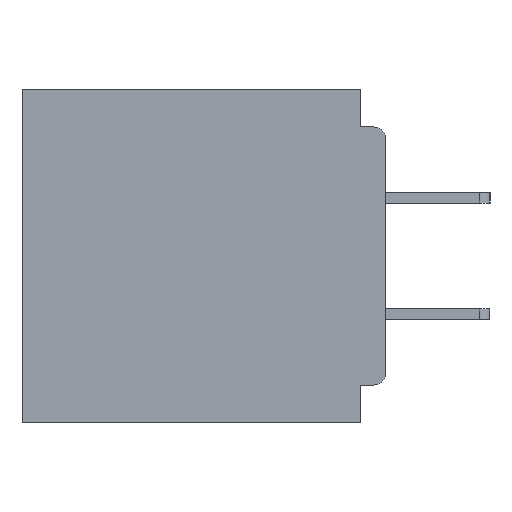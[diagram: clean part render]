
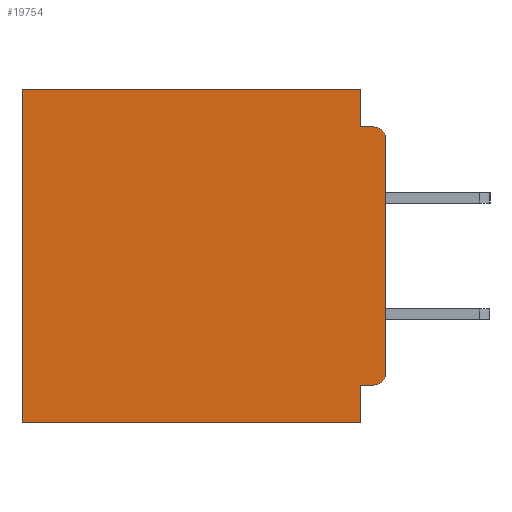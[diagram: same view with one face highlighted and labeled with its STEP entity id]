
A CAD part, left-side view. The second image highlights one B-rep face of the part: STEP entity #19754.
In plain terms, the highlighted planar face has unit normal (-1, 0, 0).
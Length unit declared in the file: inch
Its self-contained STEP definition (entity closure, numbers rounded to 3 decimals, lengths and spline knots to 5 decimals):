
#26 = VECTOR ( 'NONE', #40239, 39.37008 ) ;
#572 = CARTESIAN_POINT ( 'NONE',  ( 0.3, 0., 0. ) ) ;
#896 = CARTESIAN_POINT ( 'NONE',  ( 0.3, 0.437, -0.4 ) ) ;
#951 = CARTESIAN_POINT ( 'NONE',  ( 0.3, 0.437, -0.4 ) ) ;
#1415 = DIRECTION ( 'NONE',  ( 0., 0., -1. ) ) ;
#1472 = LINE ( 'NONE', #30982, #26 ) ;
#1840 = DIRECTION ( 'NONE',  ( -1., 0., 0. ) ) ;
#1983 = LINE ( 'NONE', #951, #49897 ) ;
#2817 = VERTEX_POINT ( 'NONE', #29447 ) ;
#5861 = EDGE_LOOP ( 'NONE', ( #54353, #28325, #51363, #54717, #31887, #22470, #36258, #59076, #18633, #49215 ) ) ;
#6317 = EDGE_CURVE ( 'NONE', #19578, #14118, #29886, .T. ) ;
#6645 = VECTOR ( 'NONE', #54614, 39.37008 ) ;
#8592 = CARTESIAN_POINT ( 'NONE',  ( 0.3, 0.437, 0. ) ) ;
#9813 = CIRCLE ( 'NONE', #55843, 0.015 ) ;
#11366 = EDGE_CURVE ( 'NONE', #14173, #22456, #1472, .T. ) ;
#14037 = VERTEX_POINT ( 'NONE', #27897 ) ;
#14118 = VERTEX_POINT ( 'NONE', #37536 ) ;
#14173 = VERTEX_POINT ( 'NONE', #51905 ) ;
#14582 = VERTEX_POINT ( 'NONE', #32452 ) ;
#15643 = VECTOR ( 'NONE', #19669, 39.37008 ) ;
#17175 = FACE_OUTER_BOUND ( 'NONE', #5861, .T. ) ;
#17502 = VECTOR ( 'NONE', #52896, 39.37008 ) ;
#18633 = ORIENTED_EDGE ( 'NONE', *, *, #27346, .F. ) ;
#19578 = VERTEX_POINT ( 'NONE', #36152 ) ;
#19669 = DIRECTION ( 'NONE',  ( 0., 1., 0. ) ) ;
#19754 = ADVANCED_FACE ( 'NONE', ( #17175 ), #38349, .F. ) ;
#19960 = DIRECTION ( 'NONE',  ( 1., 0., 0. ) ) ;
#20280 = VECTOR ( 'NONE', #44851, 39.37008 ) ;
#20535 = CARTESIAN_POINT ( 'NONE',  ( 0.3, 0., -0.4 ) ) ;
#20825 = EDGE_CURVE ( 'NONE', #14173, #14118, #9813, .T. ) ;
#21878 = CARTESIAN_POINT ( 'NONE',  ( 0.3, 0.031, 0. ) ) ;
#22235 = CARTESIAN_POINT ( 'NONE',  ( 0.3, 0., -0.045 ) ) ;
#22456 = VERTEX_POINT ( 'NONE', #36747 ) ;
#22470 = ORIENTED_EDGE ( 'NONE', *, *, #32118, .T. ) ;
#22947 = VERTEX_POINT ( 'NONE', #8592 ) ;
#23770 = DIRECTION ( 'NONE',  ( 0., 1., 0. ) ) ;
#25035 = CARTESIAN_POINT ( 'NONE',  ( 0.3, 0.031, 0. ) ) ;
#25443 = EDGE_CURVE ( 'NONE', #2817, #14582, #34043, .T. ) ;
#25725 = EDGE_CURVE ( 'NONE', #42033, #22947, #56533, .T. ) ;
#27346 = EDGE_CURVE ( 'NONE', #14037, #2817, #52623, .T. ) ;
#27897 = CARTESIAN_POINT ( 'NONE',  ( 0.3, 0.015, -0.355 ) ) ;
#28325 = ORIENTED_EDGE ( 'NONE', *, *, #20825, .T. ) ;
#28558 = EDGE_CURVE ( 'NONE', #42033, #19578, #32170, .T. ) ;
#29290 = DIRECTION ( 'NONE',  ( -1., 0., 0. ) ) ;
#29447 = CARTESIAN_POINT ( 'NONE',  ( 0.3, 0.031, -0.355 ) ) ;
#29703 = CARTESIAN_POINT ( 'NONE',  ( 0.3, 0.015, -0.06 ) ) ;
#29712 = EDGE_CURVE ( 'NONE', #14582, #36507, #29876, .T. ) ;
#29876 = LINE ( 'NONE', #20535, #17502 ) ;
#29886 = LINE ( 'NONE', #22235, #6645 ) ;
#30982 = CARTESIAN_POINT ( 'NONE',  ( 0.3, 0., -0.4 ) ) ;
#31887 = ORIENTED_EDGE ( 'NONE', *, *, #25725, .T. ) ;
#32118 = EDGE_CURVE ( 'NONE', #22947, #36507, #1983, .T. ) ;
#32170 = LINE ( 'NONE', #25035, #53879 ) ;
#32452 = CARTESIAN_POINT ( 'NONE',  ( 0.3, 0.031, -0.4 ) ) ;
#34043 = LINE ( 'NONE', #40162, #20280 ) ;
#34300 = DIRECTION ( 'NONE',  ( 0., 0., -1. ) ) ;
#34403 = AXIS2_PLACEMENT_3D ( 'NONE', #47668, #19960, #52348 ) ;
#36152 = CARTESIAN_POINT ( 'NONE',  ( 0.3, 0.031, -0.045 ) ) ;
#36258 = ORIENTED_EDGE ( 'NONE', *, *, #29712, .F. ) ;
#36507 = VERTEX_POINT ( 'NONE', #896 ) ;
#36747 = CARTESIAN_POINT ( 'NONE',  ( 0.3, 0., -0.34 ) ) ;
#37536 = CARTESIAN_POINT ( 'NONE',  ( 0.3, 0.015, -0.045 ) ) ;
#38349 = PLANE ( 'NONE',  #34403 ) ;
#40162 = CARTESIAN_POINT ( 'NONE',  ( 0.3, 0.031, -0.4 ) ) ;
#40239 = DIRECTION ( 'NONE',  ( 0., 0., -1. ) ) ;
#42033 = VERTEX_POINT ( 'NONE', #21878 ) ;
#42042 = CIRCLE ( 'NONE', #52675, 0.015 ) ;
#44851 = DIRECTION ( 'NONE',  ( 0., 0., -1. ) ) ;
#45140 = EDGE_CURVE ( 'NONE', #14037, #22456, #42042, .T. ) ;
#47370 = CARTESIAN_POINT ( 'NONE',  ( 0.3, 0., -0.355 ) ) ;
#47390 = DIRECTION ( 'NONE',  ( 0., 0., -1. ) ) ;
#47668 = CARTESIAN_POINT ( 'NONE',  ( 0.3, 0., -0.4 ) ) ;
#49215 = ORIENTED_EDGE ( 'NONE', *, *, #45140, .T. ) ;
#49897 = VECTOR ( 'NONE', #47390, 39.37008 ) ;
#51363 = ORIENTED_EDGE ( 'NONE', *, *, #6317, .F. ) ;
#51905 = CARTESIAN_POINT ( 'NONE',  ( 0.3, 0., -0.06 ) ) ;
#52348 = DIRECTION ( 'NONE',  ( 0., 0., -1. ) ) ;
#52623 = LINE ( 'NONE', #47370, #15643 ) ;
#52675 = AXIS2_PLACEMENT_3D ( 'NONE', #57064, #29290, #1415 ) ;
#52722 = DIRECTION ( 'NONE',  ( 0., 0., -1. ) ) ;
#52896 = DIRECTION ( 'NONE',  ( 0., 1., 0. ) ) ;
#53879 = VECTOR ( 'NONE', #52722, 39.37008 ) ;
#54353 = ORIENTED_EDGE ( 'NONE', *, *, #11366, .F. ) ;
#54614 = DIRECTION ( 'NONE',  ( 0., -1., 0. ) ) ;
#54717 = ORIENTED_EDGE ( 'NONE', *, *, #28558, .F. ) ;
#55046 = VECTOR ( 'NONE', #23770, 39.37008 ) ;
#55843 = AXIS2_PLACEMENT_3D ( 'NONE', #29703, #1840, #34300 ) ;
#56533 = LINE ( 'NONE', #572, #55046 ) ;
#57064 = CARTESIAN_POINT ( 'NONE',  ( 0.3, 0.015, -0.34 ) ) ;
#59076 = ORIENTED_EDGE ( 'NONE', *, *, #25443, .F. ) ;
